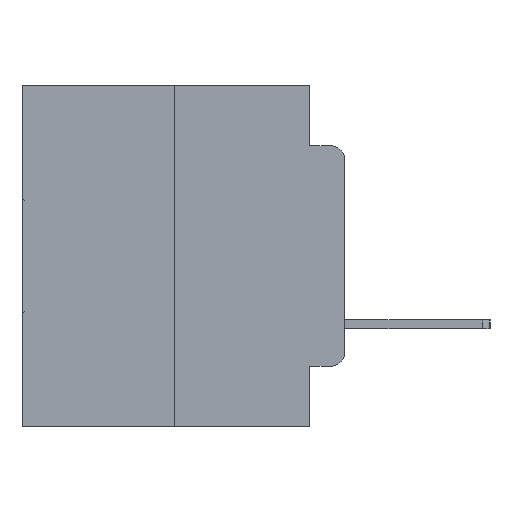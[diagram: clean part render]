
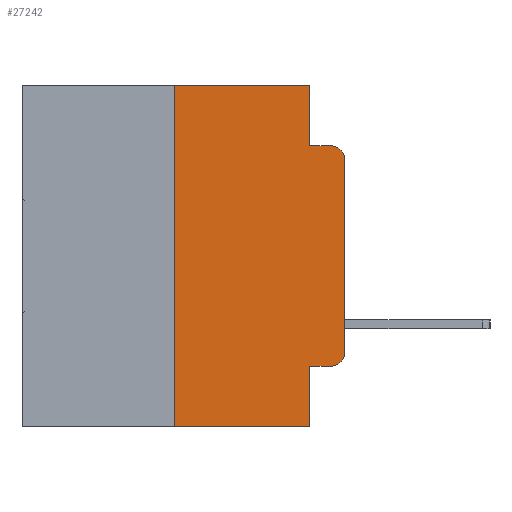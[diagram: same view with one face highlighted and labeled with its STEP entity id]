
A CAD part, left-side view. The second image highlights one B-rep face of the part: STEP entity #27242.
In plain terms, the highlighted planar face has unit normal (-1, 0, 0).
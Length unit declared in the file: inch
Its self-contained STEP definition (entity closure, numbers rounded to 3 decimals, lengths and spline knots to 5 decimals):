
#154 = VERTEX_POINT ( 'NONE', #26683 ) ;
#358 = LINE ( 'NONE', #8752, #18526 ) ;
#618 = ORIENTED_EDGE ( 'NONE', *, *, #8812, .F. ) ;
#891 = EDGE_CURVE ( 'NONE', #2366, #8552, #23342, .T. ) ;
#1251 = VERTEX_POINT ( 'NONE', #21457 ) ;
#1691 = DIRECTION ( 'NONE',  ( -1., 0., 0. ) ) ;
#1973 = FACE_OUTER_BOUND ( 'NONE', #10170, .T. ) ;
#2139 = EDGE_CURVE ( 'NONE', #154, #13105, #8181, .T. ) ;
#2216 = ORIENTED_EDGE ( 'NONE', *, *, #15185, .T. ) ;
#2366 = VERTEX_POINT ( 'NONE', #28154 ) ;
#2978 = VERTEX_POINT ( 'NONE', #16595 ) ;
#3032 = DIRECTION ( 'NONE',  ( -1., 0., 0. ) ) ;
#3217 = VECTOR ( 'NONE', #24188, 39.37008 ) ;
#3222 = LINE ( 'NONE', #12144, #21112 ) ;
#3767 = ORIENTED_EDGE ( 'NONE', *, *, #6576, .T. ) ;
#4418 = CARTESIAN_POINT ( 'NONE',  ( 0., 0.25, 0. ) ) ;
#5500 = VECTOR ( 'NONE', #9632, 39.37008 ) ;
#5609 = ORIENTED_EDGE ( 'NONE', *, *, #13226, .F. ) ;
#5785 = AXIS2_PLACEMENT_3D ( 'NONE', #17070, #3032, #19412 ) ;
#6240 = CARTESIAN_POINT ( 'NONE',  ( 0., 0.051, 0. ) ) ;
#6576 = EDGE_CURVE ( 'NONE', #24099, #154, #358, .T. ) ;
#7466 = CARTESIAN_POINT ( 'NONE',  ( 0., 0.25, 0. ) ) ;
#8133 = CARTESIAN_POINT ( 'NONE',  ( 0., 0., -0.1085 ) ) ;
#8181 = CIRCLE ( 'NONE', #26771, 0.02 ) ;
#8552 = VERTEX_POINT ( 'NONE', #4418 ) ;
#8602 = LINE ( 'NONE', #6240, #26403 ) ;
#8752 = CARTESIAN_POINT ( 'NONE',  ( 0., 0.051, -0.4115 ) ) ;
#8812 = EDGE_CURVE ( 'NONE', #8552, #1251, #9448, .T. ) ;
#9245 = ORIENTED_EDGE ( 'NONE', *, *, #27079, .F. ) ;
#9448 = LINE ( 'NONE', #21868, #3217 ) ;
#9632 = DIRECTION ( 'NONE',  ( 0., -1., 0. ) ) ;
#9732 = VERTEX_POINT ( 'NONE', #19194 ) ;
#9917 = CARTESIAN_POINT ( 'NONE',  ( 0., 0.051, -0.4115 ) ) ;
#9932 = DIRECTION ( 'NONE',  ( 0., -1., 0. ) ) ;
#10002 = CARTESIAN_POINT ( 'NONE',  ( 0., 0.473, 0. ) ) ;
#10170 = EDGE_LOOP ( 'NONE', ( #22726, #11098, #5609, #11830, #618, #26339, #2216, #9245, #3767, #22380 ) ) ;
#11098 = ORIENTED_EDGE ( 'NONE', *, *, #28457, .T. ) ;
#11830 = ORIENTED_EDGE ( 'NONE', *, *, #24383, .F. ) ;
#12144 = CARTESIAN_POINT ( 'NONE',  ( 0., 0., 0. ) ) ;
#12360 = DIRECTION ( 'NONE',  ( 0., 0., -1. ) ) ;
#12385 = VERTEX_POINT ( 'NONE', #8133 ) ;
#13105 = VERTEX_POINT ( 'NONE', #25390 ) ;
#13226 = EDGE_CURVE ( 'NONE', #2978, #9732, #24077, .T. ) ;
#13990 = CARTESIAN_POINT ( 'NONE',  ( 0., 0.051, 0. ) ) ;
#14218 = CARTESIAN_POINT ( 'NONE',  ( 0., 0.051, -0.0885 ) ) ;
#14408 = CARTESIAN_POINT ( 'NONE',  ( 0., 0.473, -0.5 ) ) ;
#15185 = EDGE_CURVE ( 'NONE', #2366, #17330, #19270, .T. ) ;
#15812 = CARTESIAN_POINT ( 'NONE',  ( 0., 0.02, -0.3915 ) ) ;
#16595 = CARTESIAN_POINT ( 'NONE',  ( 0., 0.051, -0.0885 ) ) ;
#17070 = CARTESIAN_POINT ( 'NONE',  ( 0., 0.02, -0.1085 ) ) ;
#17330 = VERTEX_POINT ( 'NONE', #18549 ) ;
#18064 = DIRECTION ( 'NONE',  ( 0., -1., 0. ) ) ;
#18192 = DIRECTION ( 'NONE',  ( 0., 0., -1. ) ) ;
#18526 = VECTOR ( 'NONE', #18064, 39.37008 ) ;
#18539 = VECTOR ( 'NONE', #9932, 39.37008 ) ;
#18549 = CARTESIAN_POINT ( 'NONE',  ( 0., 0.051, -0.5 ) ) ;
#18661 = VECTOR ( 'NONE', #26134, 39.37008 ) ;
#19178 = DIRECTION ( 'NONE',  ( 0., 0., 1. ) ) ;
#19194 = CARTESIAN_POINT ( 'NONE',  ( 0., 0.02, -0.0885 ) ) ;
#19270 = LINE ( 'NONE', #14408, #18539 ) ;
#19412 = DIRECTION ( 'NONE',  ( 0., 0., -1. ) ) ;
#21112 = VECTOR ( 'NONE', #19178, 39.37008 ) ;
#21358 = CIRCLE ( 'NONE', #5785, 0.02 ) ;
#21457 = CARTESIAN_POINT ( 'NONE',  ( 0., 0.051, 0. ) ) ;
#21868 = CARTESIAN_POINT ( 'NONE',  ( 0., 0.473, 0. ) ) ;
#22380 = ORIENTED_EDGE ( 'NONE', *, *, #2139, .T. ) ;
#22726 = ORIENTED_EDGE ( 'NONE', *, *, #26495, .T. ) ;
#23342 = LINE ( 'NONE', #7466, #18661 ) ;
#23917 = PLANE ( 'NONE',  #24273 ) ;
#24077 = LINE ( 'NONE', #14218, #5500 ) ;
#24099 = VERTEX_POINT ( 'NONE', #9917 ) ;
#24188 = DIRECTION ( 'NONE',  ( 0., -1., 0. ) ) ;
#24273 = AXIS2_PLACEMENT_3D ( 'NONE', #10002, #26240, #12360 ) ;
#24350 = LINE ( 'NONE', #13990, #29696 ) ;
#24383 = EDGE_CURVE ( 'NONE', #1251, #2978, #8602, .T. ) ;
#24833 = DIRECTION ( 'NONE',  ( 0., 0., -1. ) ) ;
#25390 = CARTESIAN_POINT ( 'NONE',  ( 0., 0., -0.3915 ) ) ;
#26134 = DIRECTION ( 'NONE',  ( 0., 0., 1. ) ) ;
#26240 = DIRECTION ( 'NONE',  ( 1., 0., 0. ) ) ;
#26339 = ORIENTED_EDGE ( 'NONE', *, *, #891, .F. ) ;
#26403 = VECTOR ( 'NONE', #24833, 39.37008 ) ;
#26495 = EDGE_CURVE ( 'NONE', #13105, #12385, #3222, .T. ) ;
#26683 = CARTESIAN_POINT ( 'NONE',  ( 0., 0.02, -0.4115 ) ) ;
#26771 = AXIS2_PLACEMENT_3D ( 'NONE', #15812, #1691, #18192 ) ;
#27079 = EDGE_CURVE ( 'NONE', #24099, #17330, #24350, .T. ) ;
#27242 = ADVANCED_FACE ( 'NONE', ( #1973 ), #23917, .F. ) ;
#28154 = CARTESIAN_POINT ( 'NONE',  ( 0., 0.25, -0.5 ) ) ;
#28457 = EDGE_CURVE ( 'NONE', #12385, #9732, #21358, .T. ) ;
#29696 = VECTOR ( 'NONE', #30216, 39.37008 ) ;
#30216 = DIRECTION ( 'NONE',  ( 0., 0., -1. ) ) ;
